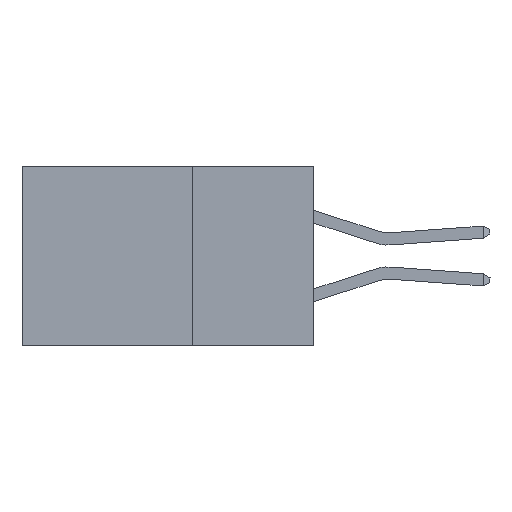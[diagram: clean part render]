
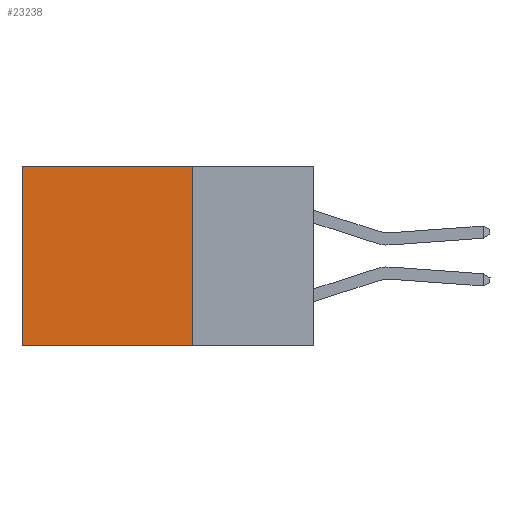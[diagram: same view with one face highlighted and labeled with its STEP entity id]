
A CAD part, left-side view. The second image highlights one B-rep face of the part: STEP entity #23238.
In plain terms, the highlighted planar face has unit normal (-1, 0, 0).
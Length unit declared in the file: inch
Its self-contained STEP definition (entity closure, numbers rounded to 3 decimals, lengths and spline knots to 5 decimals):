
#710 = LINE ( 'NONE', #38579, #20735 ) ;
#1209 = CARTESIAN_POINT ( 'NONE',  ( 0.2875, 0.6, 0. ) ) ;
#1619 = VERTEX_POINT ( 'NONE', #19015 ) ;
#4199 = DIRECTION ( 'NONE',  ( 0., 0., -1. ) ) ;
#8259 = VECTOR ( 'NONE', #27008, 39.37008 ) ;
#8999 = CARTESIAN_POINT ( 'NONE',  ( 0.2875, 0.25, 0. ) ) ;
#9662 = CARTESIAN_POINT ( 'NONE',  ( 0.2875, 0.6, 0. ) ) ;
#10347 = DIRECTION ( 'NONE',  ( 0., 1., 0. ) ) ;
#11558 = VECTOR ( 'NONE', #10347, 39.37008 ) ;
#11645 = DIRECTION ( 'NONE',  ( 1., 0., 0. ) ) ;
#12162 = EDGE_CURVE ( 'NONE', #1619, #21127, #17337, .T. ) ;
#12600 = VERTEX_POINT ( 'NONE', #15355 ) ;
#13250 = AXIS2_PLACEMENT_3D ( 'NONE', #21774, #11645, #4199 ) ;
#15355 = CARTESIAN_POINT ( 'NONE',  ( 0.2875, 0.25, 0. ) ) ;
#16476 = EDGE_LOOP ( 'NONE', ( #35353, #37707, #23090, #21859 ) ) ;
#17337 = LINE ( 'NONE', #20252, #11558 ) ;
#19015 = CARTESIAN_POINT ( 'NONE',  ( 0.2875, 0.25, -0.37 ) ) ;
#19143 = LINE ( 'NONE', #8999, #8259 ) ;
#20035 = VERTEX_POINT ( 'NONE', #1209 ) ;
#20252 = CARTESIAN_POINT ( 'NONE',  ( 0.2875, 0.25, -0.37 ) ) ;
#20735 = VECTOR ( 'NONE', #27747, 39.37008 ) ;
#21127 = VERTEX_POINT ( 'NONE', #25268 ) ;
#21774 = CARTESIAN_POINT ( 'NONE',  ( 0.2875, 0.25, 0. ) ) ;
#21859 = ORIENTED_EDGE ( 'NONE', *, *, #27837, .T. ) ;
#23090 = ORIENTED_EDGE ( 'NONE', *, *, #36574, .F. ) ;
#23238 = ADVANCED_FACE ( 'NONE', ( #35100 ), #28528, .F. ) ;
#24898 = VECTOR ( 'NONE', #26586, 39.37008 ) ;
#25268 = CARTESIAN_POINT ( 'NONE',  ( 0.2875, 0.6, -0.37 ) ) ;
#26586 = DIRECTION ( 'NONE',  ( 0., 0., -1. ) ) ;
#27008 = DIRECTION ( 'NONE',  ( 0., 0., -1. ) ) ;
#27747 = DIRECTION ( 'NONE',  ( 0., 1., 0. ) ) ;
#27837 = EDGE_CURVE ( 'NONE', #12600, #20035, #710, .T. ) ;
#28528 = PLANE ( 'NONE',  #13250 ) ;
#35100 = FACE_OUTER_BOUND ( 'NONE', #16476, .T. ) ;
#35353 = ORIENTED_EDGE ( 'NONE', *, *, #37824, .T. ) ;
#36574 = EDGE_CURVE ( 'NONE', #12600, #1619, #19143, .T. ) ;
#37707 = ORIENTED_EDGE ( 'NONE', *, *, #12162, .F. ) ;
#37824 = EDGE_CURVE ( 'NONE', #20035, #21127, #40336, .T. ) ;
#38579 = CARTESIAN_POINT ( 'NONE',  ( 0.2875, 0.25, 0. ) ) ;
#40336 = LINE ( 'NONE', #9662, #24898 ) ;
